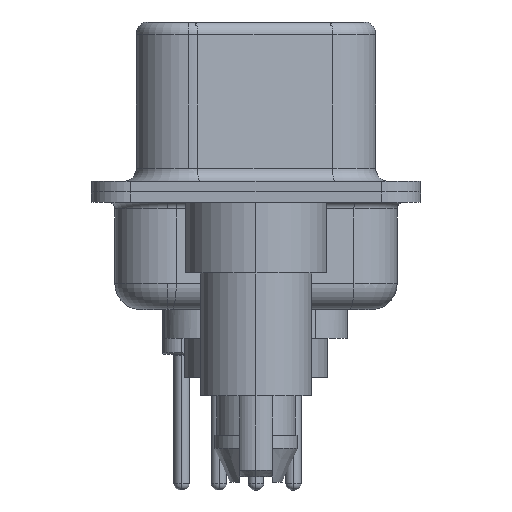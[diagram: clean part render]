
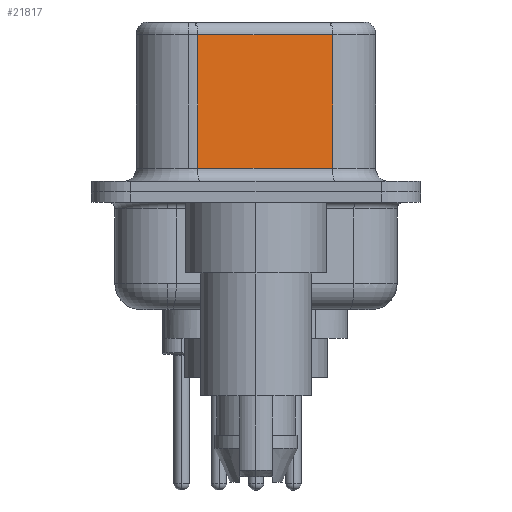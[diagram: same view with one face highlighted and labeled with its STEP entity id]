
A CAD part, left-side view. The second image highlights one B-rep face of the part: STEP entity #21817.
In plain terms, the highlighted planar face has unit normal (-0.985, -0.174, 0).
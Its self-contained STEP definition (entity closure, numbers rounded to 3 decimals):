
#544 = ORIENTED_EDGE ( 'NONE', *, *, #4433, .T. ) ;
#721 = ORIENTED_EDGE ( 'NONE', *, *, #12791, .F. ) ;
#1054 = FACE_OUTER_BOUND ( 'NONE', #3561, .T. ) ;
#2165 = EDGE_CURVE ( 'NONE', #8089, #23124, #8876, .T. ) ;
#2188 = VERTEX_POINT ( 'NONE', #9162 ) ;
#2781 = VECTOR ( 'NONE', #8139, 1000. ) ;
#3561 = EDGE_LOOP ( 'NONE', ( #721, #8153, #6250, #544 ) ) ;
#4433 = EDGE_CURVE ( 'NONE', #23124, #2188, #8528, .T. ) ;
#6250 = ORIENTED_EDGE ( 'NONE', *, *, #2165, .T. ) ;
#7351 = VECTOR ( 'NONE', #10163, 1000. ) ;
#8089 = VERTEX_POINT ( 'NONE', #14983 ) ;
#8139 = DIRECTION ( 'NONE',  ( 0.174, -0.985, 0. ) ) ;
#8153 = ORIENTED_EDGE ( 'NONE', *, *, #11179, .T. ) ;
#8528 = LINE ( 'NONE', #9800, #2781 ) ;
#8876 = LINE ( 'NONE', #9301, #14109 ) ;
#9162 = CARTESIAN_POINT ( 'NONE',  ( 4.58, -2.927, 0.9 ) ) ;
#9301 = CARTESIAN_POINT ( 'NONE',  ( 3.67, 2.233, 6.52 ) ) ;
#9559 = DIRECTION ( 'NONE',  ( 0., 0., -1. ) ) ;
#9657 = DIRECTION ( 'NONE',  ( -0.174, 0.985, 0. ) ) ;
#9800 = CARTESIAN_POINT ( 'NONE',  ( 4.58, -2.927, 0.9 ) ) ;
#10163 = DIRECTION ( 'NONE',  ( 0., 0., -1. ) ) ;
#11179 = EDGE_CURVE ( 'NONE', #24842, #8089, #11369, .T. ) ;
#11369 = LINE ( 'NONE', #24216, #21844 ) ;
#12398 = DIRECTION ( 'NONE',  ( -0.174, 0.985, 0. ) ) ;
#12791 = EDGE_CURVE ( 'NONE', #24842, #2188, #17170, .T. ) ;
#14109 = VECTOR ( 'NONE', #9559, 1000. ) ;
#14983 = CARTESIAN_POINT ( 'NONE',  ( 3.67, 2.233, 6.02 ) ) ;
#16309 = CARTESIAN_POINT ( 'NONE',  ( 3.67, 2.233, 0.9 ) ) ;
#17170 = LINE ( 'NONE', #21976, #7351 ) ;
#17515 = CARTESIAN_POINT ( 'NONE',  ( 4.58, -2.927, 6.52 ) ) ;
#17648 = AXIS2_PLACEMENT_3D ( 'NONE', #17515, #21457, #9657 ) ;
#21457 = DIRECTION ( 'NONE',  ( 0.985, 0.174, 0. ) ) ;
#21800 = CARTESIAN_POINT ( 'NONE',  ( 4.58, -2.927, 6.02 ) ) ;
#21817 = ADVANCED_FACE ( 'NONE', ( #1054 ), #25396, .F. ) ;
#21844 = VECTOR ( 'NONE', #12398, 1000. ) ;
#21976 = CARTESIAN_POINT ( 'NONE',  ( 4.58, -2.927, 6.52 ) ) ;
#23124 = VERTEX_POINT ( 'NONE', #16309 ) ;
#24216 = CARTESIAN_POINT ( 'NONE',  ( 4.58, -2.927, 6.02 ) ) ;
#24842 = VERTEX_POINT ( 'NONE', #21800 ) ;
#25396 = PLANE ( 'NONE',  #17648 ) ;
